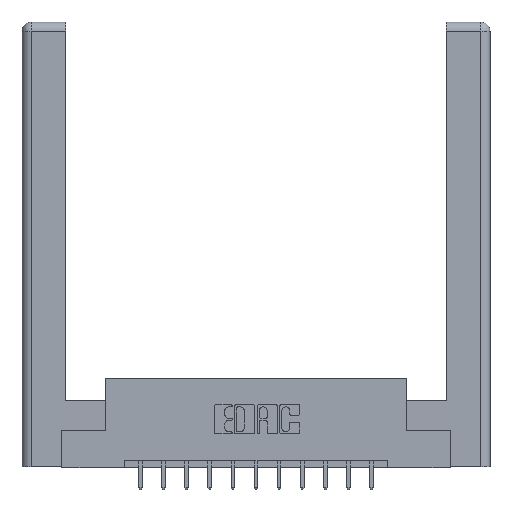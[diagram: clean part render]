
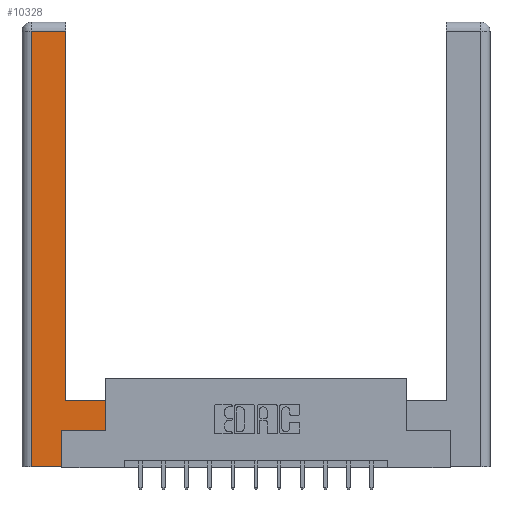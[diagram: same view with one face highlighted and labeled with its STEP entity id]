
A CAD part, top view. The second image highlights one B-rep face of the part: STEP entity #10328.
In plain terms, the highlighted planar face has unit normal (0, 0, 1).
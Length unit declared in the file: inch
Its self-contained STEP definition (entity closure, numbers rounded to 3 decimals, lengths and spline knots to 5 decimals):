
#36 = VECTOR ( 'NONE', #10459, 39.37008 ) ;
#186 = VERTEX_POINT ( 'NONE', #4448 ) ;
#379 = LINE ( 'NONE', #1256, #14503 ) ;
#441 = ORIENTED_EDGE ( 'NONE', *, *, #8353, .T. ) ;
#664 = CARTESIAN_POINT ( 'NONE',  ( 0.295, 3., 0. ) ) ;
#669 = DIRECTION ( 'NONE',  ( -1., 0., 0. ) ) ;
#924 = VECTOR ( 'NONE', #13758, 39.37008 ) ;
#1011 = VERTEX_POINT ( 'NONE', #8379 ) ;
#1016 = EDGE_CURVE ( 'NONE', #14617, #1140, #9654, .T. ) ;
#1140 = VERTEX_POINT ( 'NONE', #9366 ) ;
#1162 = CARTESIAN_POINT ( 'NONE',  ( 0.265, 0., 0. ) ) ;
#1202 = DIRECTION ( 'NONE',  ( 1., 0., 0. ) ) ;
#1256 = CARTESIAN_POINT ( 'NONE',  ( 0.565, 0.245, 0. ) ) ;
#1584 = VERTEX_POINT ( 'NONE', #1162 ) ;
#1897 = DIRECTION ( 'NONE',  ( 0., -1., 0. ) ) ;
#2374 = CARTESIAN_POINT ( 'NONE',  ( 0.295, 2.94, 0. ) ) ;
#2553 = DIRECTION ( 'NONE',  ( 1., 0., 0. ) ) ;
#2632 = VECTOR ( 'NONE', #669, 39.37008 ) ;
#2808 = VECTOR ( 'NONE', #1897, 39.37008 ) ;
#3283 = EDGE_CURVE ( 'NONE', #1140, #4094, #14717, .T. ) ;
#3910 = EDGE_CURVE ( 'NONE', #14938, #1011, #379, .T. ) ;
#4094 = VERTEX_POINT ( 'NONE', #12234 ) ;
#4232 = DIRECTION ( 'NONE',  ( -1., 0., 0. ) ) ;
#4448 = CARTESIAN_POINT ( 'NONE',  ( 0.295, 0.45, 0. ) ) ;
#4685 = EDGE_CURVE ( 'NONE', #186, #14617, #13013, .T. ) ;
#4764 = ORIENTED_EDGE ( 'NONE', *, *, #1016, .T. ) ;
#4862 = ORIENTED_EDGE ( 'NONE', *, *, #14916, .T. ) ;
#4952 = VECTOR ( 'NONE', #10046, 39.37008 ) ;
#4978 = CARTESIAN_POINT ( 'NONE',  ( 0.565, 0.45, 0. ) ) ;
#5377 = DIRECTION ( 'NONE',  ( 0., 0., -1. ) ) ;
#5460 = CARTESIAN_POINT ( 'NONE',  ( 0.265, 0., 0. ) ) ;
#5492 = EDGE_CURVE ( 'NONE', #4094, #1584, #10619, .T. ) ;
#5548 = AXIS2_PLACEMENT_3D ( 'NONE', #7729, #5377, #4232 ) ;
#6042 = DIRECTION ( 'NONE',  ( -1., 0., 0. ) ) ;
#6081 = ORIENTED_EDGE ( 'NONE', *, *, #7728, .T. ) ;
#6614 = PLANE ( 'NONE',  #5548 ) ;
#6689 = LINE ( 'NONE', #10369, #36 ) ;
#7267 = FACE_OUTER_BOUND ( 'NONE', #14011, .T. ) ;
#7497 = CARTESIAN_POINT ( 'NONE',  ( 0.265, 0.245, 0. ) ) ;
#7717 = CARTESIAN_POINT ( 'NONE',  ( 0.295, 0.45, 0. ) ) ;
#7728 = EDGE_CURVE ( 'NONE', #1011, #13514, #6689, .T. ) ;
#7729 = CARTESIAN_POINT ( 'NONE',  ( 0., 0., 0. ) ) ;
#7734 = ORIENTED_EDGE ( 'NONE', *, *, #4685, .T. ) ;
#8353 = EDGE_CURVE ( 'NONE', #1584, #14938, #11952, .T. ) ;
#8379 = CARTESIAN_POINT ( 'NONE',  ( 0.565, 0.245, 0. ) ) ;
#8487 = ORIENTED_EDGE ( 'NONE', *, *, #3283, .T. ) ;
#9366 = CARTESIAN_POINT ( 'NONE',  ( 0.0615, 2.94, 0. ) ) ;
#9471 = VECTOR ( 'NONE', #6042, 39.37008 ) ;
#9654 = LINE ( 'NONE', #11857, #9471 ) ;
#9713 = VECTOR ( 'NONE', #1202, 39.37008 ) ;
#9810 = ORIENTED_EDGE ( 'NONE', *, *, #5492, .T. ) ;
#10046 = DIRECTION ( 'NONE',  ( 0., 1., 0. ) ) ;
#10304 = CARTESIAN_POINT ( 'NONE',  ( 0.265, 0.245, 0. ) ) ;
#10328 = ADVANCED_FACE ( 'NONE', ( #7267 ), #6614, .F. ) ;
#10369 = CARTESIAN_POINT ( 'NONE',  ( 0.565, 0.45, 0. ) ) ;
#10448 = ORIENTED_EDGE ( 'NONE', *, *, #3910, .T. ) ;
#10459 = DIRECTION ( 'NONE',  ( 0., 1., 0. ) ) ;
#10619 = LINE ( 'NONE', #5460, #9713 ) ;
#11857 = CARTESIAN_POINT ( 'NONE',  ( 0.0615, 2.94, 0. ) ) ;
#11952 = LINE ( 'NONE', #7497, #924 ) ;
#12234 = CARTESIAN_POINT ( 'NONE',  ( 0.0615, 0., 0. ) ) ;
#13013 = LINE ( 'NONE', #664, #4952 ) ;
#13514 = VERTEX_POINT ( 'NONE', #4978 ) ;
#13616 = LINE ( 'NONE', #7717, #2632 ) ;
#13758 = DIRECTION ( 'NONE',  ( 0., 1., 0. ) ) ;
#14011 = EDGE_LOOP ( 'NONE', ( #7734, #4764, #8487, #9810, #441, #10448, #6081, #4862 ) ) ;
#14503 = VECTOR ( 'NONE', #2553, 39.37008 ) ;
#14617 = VERTEX_POINT ( 'NONE', #2374 ) ;
#14717 = LINE ( 'NONE', #14927, #2808 ) ;
#14916 = EDGE_CURVE ( 'NONE', #13514, #186, #13616, .T. ) ;
#14927 = CARTESIAN_POINT ( 'NONE',  ( 0.0615, 0., 0. ) ) ;
#14938 = VERTEX_POINT ( 'NONE', #10304 ) ;
